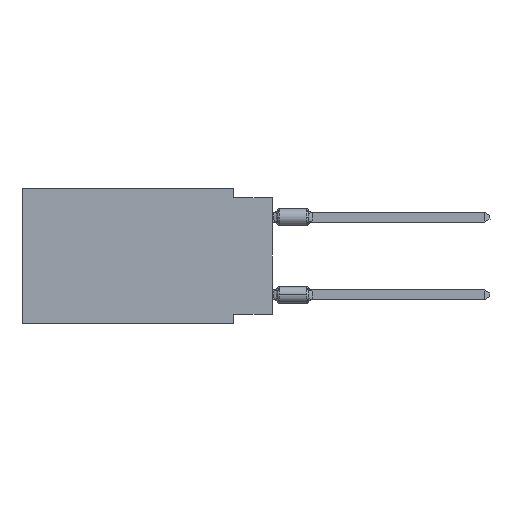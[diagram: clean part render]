
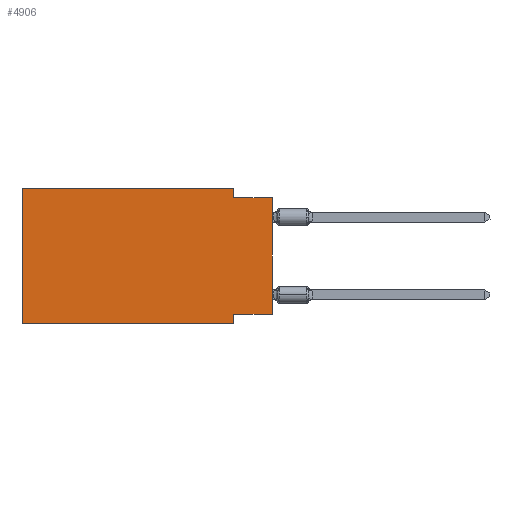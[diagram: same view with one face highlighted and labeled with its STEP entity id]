
A CAD part, left-side view. The second image highlights one B-rep face of the part: STEP entity #4906.
In plain terms, the highlighted planar face has unit normal (-1, 0, 0).
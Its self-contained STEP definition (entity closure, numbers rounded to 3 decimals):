
#319 = LINE ( 'NONE', #5517, #9291 ) ;
#362 = EDGE_CURVE ( 'NONE', #17973, #20747, #14701, .T. ) ;
#548 = DIRECTION ( 'NONE',  ( 0., 1., 0. ) ) ;
#668 = LINE ( 'NONE', #11052, #18058 ) ;
#806 = CARTESIAN_POINT ( 'NONE',  ( 0., 16.383, 0. ) ) ;
#881 = LINE ( 'NONE', #1224, #8382 ) ;
#1216 = EDGE_CURVE ( 'NONE', #1851, #19766, #12054, .T. ) ;
#1224 = CARTESIAN_POINT ( 'NONE',  ( 0., 16.383, 0. ) ) ;
#1851 = VERTEX_POINT ( 'NONE', #6032 ) ;
#2641 = CARTESIAN_POINT ( 'NONE',  ( 0., 2.54, -8.89 ) ) ;
#4021 = EDGE_CURVE ( 'NONE', #17973, #8191, #668, .T. ) ;
#4348 = CARTESIAN_POINT ( 'NONE',  ( 0., 0., 0. ) ) ;
#4683 = DIRECTION ( 'NONE',  ( 0., -1., 0. ) ) ;
#4906 = ADVANCED_FACE ( 'NONE', ( #6925 ), #13822, .F. ) ;
#5517 = CARTESIAN_POINT ( 'NONE',  ( 0., 0., -0.635 ) ) ;
#5841 = EDGE_CURVE ( 'NONE', #21873, #12855, #21583, .T. ) ;
#6032 = CARTESIAN_POINT ( 'NONE',  ( 0., 2.54, 0. ) ) ;
#6452 = VECTOR ( 'NONE', #20673, 1000. ) ;
#6761 = VERTEX_POINT ( 'NONE', #2641 ) ;
#6821 = DIRECTION ( 'NONE',  ( 0., -1., 0. ) ) ;
#6857 = ORIENTED_EDGE ( 'NONE', *, *, #4021, .F. ) ;
#6925 = FACE_OUTER_BOUND ( 'NONE', #11255, .T. ) ;
#8191 = VERTEX_POINT ( 'NONE', #21835 ) ;
#8382 = VECTOR ( 'NONE', #4683, 1000. ) ;
#8522 = DIRECTION ( 'NONE',  ( 0., 0., -1. ) ) ;
#9291 = VECTOR ( 'NONE', #6821, 1000. ) ;
#9504 = ORIENTED_EDGE ( 'NONE', *, *, #16239, .F. ) ;
#9722 = CARTESIAN_POINT ( 'NONE',  ( 0., 16.383, -8.89 ) ) ;
#9792 = DIRECTION ( 'NONE',  ( 0., -1., 0. ) ) ;
#10465 = ORIENTED_EDGE ( 'NONE', *, *, #13608, .F. ) ;
#10772 = DIRECTION ( 'NONE',  ( 0., 0., 1. ) ) ;
#11052 = CARTESIAN_POINT ( 'NONE',  ( 0., 0., -8.255 ) ) ;
#11255 = EDGE_LOOP ( 'NONE', ( #21892, #20995, #20657, #9504, #12834, #13117, #10465, #6857 ) ) ;
#12054 = LINE ( 'NONE', #18616, #6452 ) ;
#12429 = DIRECTION ( 'NONE',  ( 0., 0., 1. ) ) ;
#12834 = ORIENTED_EDGE ( 'NONE', *, *, #5841, .F. ) ;
#12855 = VERTEX_POINT ( 'NONE', #806 ) ;
#13117 = ORIENTED_EDGE ( 'NONE', *, *, #14551, .T. ) ;
#13608 = EDGE_CURVE ( 'NONE', #8191, #6761, #14665, .T. ) ;
#13822 = PLANE ( 'NONE',  #14400 ) ;
#13942 = DIRECTION ( 'NONE',  ( 1., 0., 0. ) ) ;
#14400 = AXIS2_PLACEMENT_3D ( 'NONE', #18580, #13942, #8522 ) ;
#14442 = CARTESIAN_POINT ( 'NONE',  ( 0., 16.383, 0. ) ) ;
#14551 = EDGE_CURVE ( 'NONE', #21873, #6761, #20582, .T. ) ;
#14665 = LINE ( 'NONE', #21689, #21960 ) ;
#14701 = LINE ( 'NONE', #4348, #18888 ) ;
#15206 = CARTESIAN_POINT ( 'NONE',  ( 0., 2.54, -0.635 ) ) ;
#15889 = VECTOR ( 'NONE', #10772, 1000. ) ;
#16239 = EDGE_CURVE ( 'NONE', #12855, #1851, #881, .T. ) ;
#17973 = VERTEX_POINT ( 'NONE', #18227 ) ;
#18040 = CARTESIAN_POINT ( 'NONE',  ( 0., 0., -0.635 ) ) ;
#18058 = VECTOR ( 'NONE', #548, 1000. ) ;
#18227 = CARTESIAN_POINT ( 'NONE',  ( 0., 0., -8.255 ) ) ;
#18580 = CARTESIAN_POINT ( 'NONE',  ( 0., 16.383, 0. ) ) ;
#18616 = CARTESIAN_POINT ( 'NONE',  ( 0., 2.54, 0. ) ) ;
#18842 = CARTESIAN_POINT ( 'NONE',  ( 0., 16.383, -8.89 ) ) ;
#18888 = VECTOR ( 'NONE', #12429, 1000. ) ;
#19766 = VERTEX_POINT ( 'NONE', #15206 ) ;
#19940 = DIRECTION ( 'NONE',  ( 0., 0., -1. ) ) ;
#20083 = VECTOR ( 'NONE', #9792, 1000. ) ;
#20582 = LINE ( 'NONE', #18842, #20083 ) ;
#20657 = ORIENTED_EDGE ( 'NONE', *, *, #1216, .F. ) ;
#20673 = DIRECTION ( 'NONE',  ( 0., 0., -1. ) ) ;
#20747 = VERTEX_POINT ( 'NONE', #18040 ) ;
#20995 = ORIENTED_EDGE ( 'NONE', *, *, #21945, .F. ) ;
#21583 = LINE ( 'NONE', #14442, #15889 ) ;
#21689 = CARTESIAN_POINT ( 'NONE',  ( 0., 2.54, -8.89 ) ) ;
#21835 = CARTESIAN_POINT ( 'NONE',  ( 0., 2.54, -8.255 ) ) ;
#21873 = VERTEX_POINT ( 'NONE', #9722 ) ;
#21892 = ORIENTED_EDGE ( 'NONE', *, *, #362, .T. ) ;
#21945 = EDGE_CURVE ( 'NONE', #19766, #20747, #319, .T. ) ;
#21960 = VECTOR ( 'NONE', #19940, 1000. ) ;
